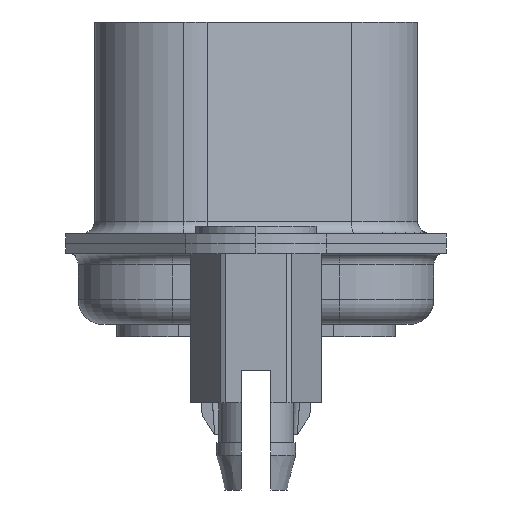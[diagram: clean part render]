
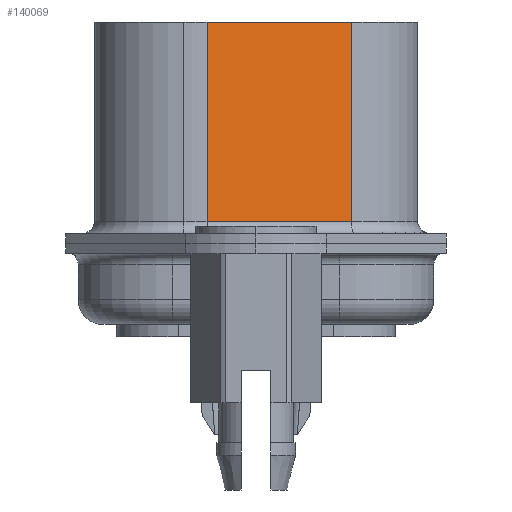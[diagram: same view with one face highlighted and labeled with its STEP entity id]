
A CAD part, left-side view. The second image highlights one B-rep face of the part: STEP entity #140069.
In plain terms, the highlighted planar face has unit normal (-0.966, -0.259, 0).
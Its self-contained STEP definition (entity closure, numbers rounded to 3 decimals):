
#512 = VECTOR ( 'NONE', #150713, 1000. ) ;
#919 = ORIENTED_EDGE ( 'NONE', *, *, #77121, .T. ) ;
#3363 = CARTESIAN_POINT ( 'NONE',  ( 6.467, -3.832, 9.3 ) ) ;
#7825 = LINE ( 'NONE', #154711, #11979 ) ;
#11979 = VECTOR ( 'NONE', #141656, 1000. ) ;
#27657 = EDGE_LOOP ( 'NONE', ( #919, #61363, #151448, #119501 ) ) ;
#29910 = LINE ( 'NONE', #68160, #512 ) ;
#38294 = CARTESIAN_POINT ( 'NONE',  ( 4.913, 1.968, 1.3 ) ) ;
#46000 = VECTOR ( 'NONE', #118961, 1000. ) ;
#53794 = CARTESIAN_POINT ( 'NONE',  ( 4.913, 1.968, 9.3 ) ) ;
#60147 = PLANE ( 'NONE',  #151726 ) ;
#61363 = ORIENTED_EDGE ( 'NONE', *, *, #107014, .T. ) ;
#62739 = DIRECTION ( 'NONE',  ( 0.966, 0.259, 0. ) ) ;
#68160 = CARTESIAN_POINT ( 'NONE',  ( 6.467, -3.832, 9.3 ) ) ;
#68669 = EDGE_CURVE ( 'NONE', #95734, #119105, #147682, .T. ) ;
#70247 = DIRECTION ( 'NONE',  ( 0.259, -0.966, 0. ) ) ;
#77121 = EDGE_CURVE ( 'NONE', #95734, #148884, #7825, .T. ) ;
#87932 = FACE_OUTER_BOUND ( 'NONE', #27657, .T. ) ;
#95734 = VERTEX_POINT ( 'NONE', #53794 ) ;
#100013 = EDGE_CURVE ( 'NONE', #119105, #109174, #29910, .T. ) ;
#105674 = CARTESIAN_POINT ( 'NONE',  ( 6.467, -3.832, 9.3 ) ) ;
#106760 = CARTESIAN_POINT ( 'NONE',  ( 6.467, -3.832, 1.3 ) ) ;
#107014 = EDGE_CURVE ( 'NONE', #148884, #109174, #118112, .T. ) ;
#109174 = VERTEX_POINT ( 'NONE', #135906 ) ;
#113171 = DIRECTION ( 'NONE',  ( -0.259, 0.966, 0. ) ) ;
#118112 = LINE ( 'NONE', #106760, #46000 ) ;
#118961 = DIRECTION ( 'NONE',  ( 0.259, -0.966, 0. ) ) ;
#119105 = VERTEX_POINT ( 'NONE', #105674 ) ;
#119501 = ORIENTED_EDGE ( 'NONE', *, *, #68669, .F. ) ;
#135906 = CARTESIAN_POINT ( 'NONE',  ( 6.467, -3.832, 1.3 ) ) ;
#140069 = ADVANCED_FACE ( 'NONE', ( #87932 ), #60147, .F. ) ;
#140997 = CARTESIAN_POINT ( 'NONE',  ( 6.467, -3.832, 9.3 ) ) ;
#141656 = DIRECTION ( 'NONE',  ( 0., 0., -1. ) ) ;
#147682 = LINE ( 'NONE', #3363, #168841 ) ;
#148884 = VERTEX_POINT ( 'NONE', #38294 ) ;
#150713 = DIRECTION ( 'NONE',  ( 0., 0., -1. ) ) ;
#151448 = ORIENTED_EDGE ( 'NONE', *, *, #100013, .F. ) ;
#151726 = AXIS2_PLACEMENT_3D ( 'NONE', #140997, #62739, #113171 ) ;
#154711 = CARTESIAN_POINT ( 'NONE',  ( 4.913, 1.968, 9.3 ) ) ;
#168841 = VECTOR ( 'NONE', #70247, 1000. ) ;
